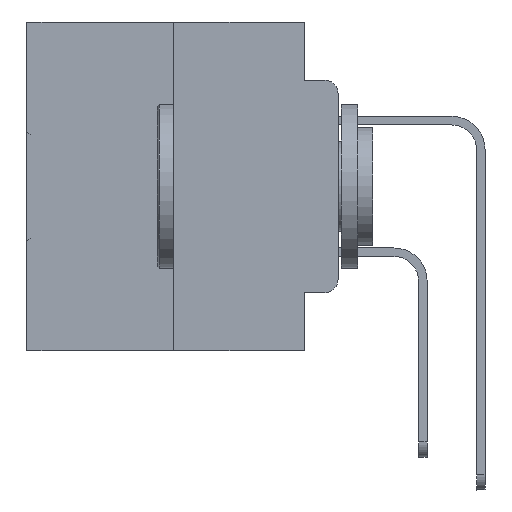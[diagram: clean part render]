
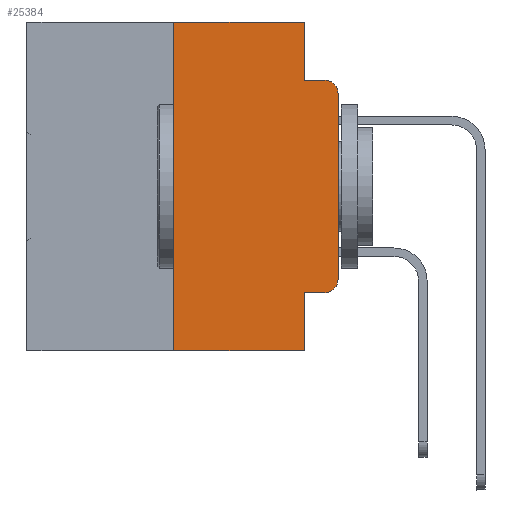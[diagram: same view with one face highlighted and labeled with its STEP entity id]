
A CAD part, left-side view. The second image highlights one B-rep face of the part: STEP entity #25384.
In plain terms, the highlighted planar face has unit normal (-1, 0, 0).
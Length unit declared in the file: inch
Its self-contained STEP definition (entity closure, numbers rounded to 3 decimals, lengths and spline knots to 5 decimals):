
#387 = EDGE_CURVE ( 'NONE', #26988, #10867, #28677, .T. ) ;
#874 = VERTEX_POINT ( 'NONE', #12031 ) ;
#957 = VERTEX_POINT ( 'NONE', #18061 ) ;
#1129 = LINE ( 'NONE', #18520, #29173 ) ;
#1601 = AXIS2_PLACEMENT_3D ( 'NONE', #15906, #8538, #18568 ) ;
#1758 = LINE ( 'NONE', #33445, #22099 ) ;
#2302 = CIRCLE ( 'NONE', #1601, 0.02 ) ;
#2676 = AXIS2_PLACEMENT_3D ( 'NONE', #10704, #29052, #13396 ) ;
#3397 = DIRECTION ( 'NONE',  ( 0., 0., 1. ) ) ;
#4855 = ORIENTED_EDGE ( 'NONE', *, *, #31710, .T. ) ;
#5334 = ORIENTED_EDGE ( 'NONE', *, *, #7924, .F. ) ;
#5744 = VERTEX_POINT ( 'NONE', #31381 ) ;
#6719 = DIRECTION ( 'NONE',  ( 0., 0., -1. ) ) ;
#6779 = ORIENTED_EDGE ( 'NONE', *, *, #32623, .T. ) ;
#6815 = VECTOR ( 'NONE', #6719, 39.37008 ) ;
#7924 = EDGE_CURVE ( 'NONE', #8188, #26548, #21773, .T. ) ;
#8188 = VERTEX_POINT ( 'NONE', #21131 ) ;
#8538 = DIRECTION ( 'NONE',  ( -1., 0., 0. ) ) ;
#8573 = LINE ( 'NONE', #29639, #21859 ) ;
#9267 = CARTESIAN_POINT ( 'NONE',  ( 0., 0.02, -0.0885 ) ) ;
#10468 = CARTESIAN_POINT ( 'NONE',  ( 0., 0.051, -0.0885 ) ) ;
#10704 = CARTESIAN_POINT ( 'NONE',  ( 0., 0.02, -0.1085 ) ) ;
#10867 = VERTEX_POINT ( 'NONE', #9267 ) ;
#12031 = CARTESIAN_POINT ( 'NONE',  ( 0., 0.25, 0. ) ) ;
#12045 = DIRECTION ( 'NONE',  ( 1., 0., 0. ) ) ;
#12969 = ORIENTED_EDGE ( 'NONE', *, *, #31514, .F. ) ;
#13012 = VECTOR ( 'NONE', #19924, 39.37008 ) ;
#13396 = DIRECTION ( 'NONE',  ( 0., 0., -1. ) ) ;
#14605 = CARTESIAN_POINT ( 'NONE',  ( 0., 0.051, -0.4115 ) ) ;
#14668 = EDGE_CURVE ( 'NONE', #957, #10867, #16752, .T. ) ;
#14859 = CARTESIAN_POINT ( 'NONE',  ( 0., 0.051, -0.5 ) ) ;
#14868 = VECTOR ( 'NONE', #3397, 39.37008 ) ;
#15863 = ORIENTED_EDGE ( 'NONE', *, *, #22875, .F. ) ;
#15906 = CARTESIAN_POINT ( 'NONE',  ( 0., 0.02, -0.3915 ) ) ;
#16551 = VERTEX_POINT ( 'NONE', #18836 ) ;
#16615 = CARTESIAN_POINT ( 'NONE',  ( 0., 0.473, -0.5 ) ) ;
#16650 = DIRECTION ( 'NONE',  ( 0., 0., -1. ) ) ;
#16752 = CIRCLE ( 'NONE', #2676, 0.02 ) ;
#17585 = VERTEX_POINT ( 'NONE', #19192 ) ;
#18061 = CARTESIAN_POINT ( 'NONE',  ( 0., 0., -0.1085 ) ) ;
#18520 = CARTESIAN_POINT ( 'NONE',  ( 0., 0.25, 0. ) ) ;
#18549 = ORIENTED_EDGE ( 'NONE', *, *, #20430, .T. ) ;
#18568 = DIRECTION ( 'NONE',  ( 0., 0., -1. ) ) ;
#18836 = CARTESIAN_POINT ( 'NONE',  ( 0., 0., -0.3915 ) ) ;
#19192 = CARTESIAN_POINT ( 'NONE',  ( 0., 0.25, -0.5 ) ) ;
#19249 = LINE ( 'NONE', #16615, #32246 ) ;
#19924 = DIRECTION ( 'NONE',  ( 0., -1., 0. ) ) ;
#20380 = DIRECTION ( 'NONE',  ( 0., -1., 0. ) ) ;
#20430 = EDGE_CURVE ( 'NONE', #8188, #27136, #33077, .T. ) ;
#21131 = CARTESIAN_POINT ( 'NONE',  ( 0., 0.051, -0.4115 ) ) ;
#21160 = DIRECTION ( 'NONE',  ( 0., 0., 1. ) ) ;
#21773 = LINE ( 'NONE', #22669, #6815 ) ;
#21780 = VECTOR ( 'NONE', #33018, 39.37008 ) ;
#21859 = VECTOR ( 'NONE', #16650, 39.37008 ) ;
#21908 = DIRECTION ( 'NONE',  ( 0., -1., 0. ) ) ;
#21944 = CARTESIAN_POINT ( 'NONE',  ( 0., 0., 0. ) ) ;
#22099 = VECTOR ( 'NONE', #20380, 39.37008 ) ;
#22256 = ORIENTED_EDGE ( 'NONE', *, *, #34060, .T. ) ;
#22555 = CARTESIAN_POINT ( 'NONE',  ( 0., 0.02, -0.4115 ) ) ;
#22669 = CARTESIAN_POINT ( 'NONE',  ( 0., 0.051, 0. ) ) ;
#22875 = EDGE_CURVE ( 'NONE', #5744, #26988, #8573, .T. ) ;
#25384 = ADVANCED_FACE ( 'NONE', ( #33466 ), #32866, .F. ) ;
#25918 = ORIENTED_EDGE ( 'NONE', *, *, #387, .F. ) ;
#26338 = ORIENTED_EDGE ( 'NONE', *, *, #14668, .T. ) ;
#26548 = VERTEX_POINT ( 'NONE', #14859 ) ;
#26988 = VERTEX_POINT ( 'NONE', #32282 ) ;
#27136 = VERTEX_POINT ( 'NONE', #22555 ) ;
#27546 = AXIS2_PLACEMENT_3D ( 'NONE', #27733, #12045, #30344 ) ;
#27733 = CARTESIAN_POINT ( 'NONE',  ( 0., 0.473, 0. ) ) ;
#28528 = EDGE_CURVE ( 'NONE', #874, #5744, #1758, .T. ) ;
#28677 = LINE ( 'NONE', #10468, #21780 ) ;
#29052 = DIRECTION ( 'NONE',  ( -1., 0., 0. ) ) ;
#29173 = VECTOR ( 'NONE', #21160, 39.37008 ) ;
#29558 = LINE ( 'NONE', #21944, #14868 ) ;
#29639 = CARTESIAN_POINT ( 'NONE',  ( 0., 0.051, 0. ) ) ;
#30330 = EDGE_LOOP ( 'NONE', ( #4855, #26338, #25918, #15863, #33025, #12969, #22256, #5334, #18549, #6779 ) ) ;
#30344 = DIRECTION ( 'NONE',  ( 0., 0., -1. ) ) ;
#31381 = CARTESIAN_POINT ( 'NONE',  ( 0., 0.051, 0. ) ) ;
#31514 = EDGE_CURVE ( 'NONE', #17585, #874, #1129, .T. ) ;
#31710 = EDGE_CURVE ( 'NONE', #16551, #957, #29558, .T. ) ;
#32246 = VECTOR ( 'NONE', #21908, 39.37008 ) ;
#32282 = CARTESIAN_POINT ( 'NONE',  ( 0., 0.051, -0.0885 ) ) ;
#32623 = EDGE_CURVE ( 'NONE', #27136, #16551, #2302, .T. ) ;
#32866 = PLANE ( 'NONE',  #27546 ) ;
#33018 = DIRECTION ( 'NONE',  ( 0., -1., 0. ) ) ;
#33025 = ORIENTED_EDGE ( 'NONE', *, *, #28528, .F. ) ;
#33077 = LINE ( 'NONE', #14605, #13012 ) ;
#33445 = CARTESIAN_POINT ( 'NONE',  ( 0., 0.473, 0. ) ) ;
#33466 = FACE_OUTER_BOUND ( 'NONE', #30330, .T. ) ;
#34060 = EDGE_CURVE ( 'NONE', #17585, #26548, #19249, .T. ) ;
